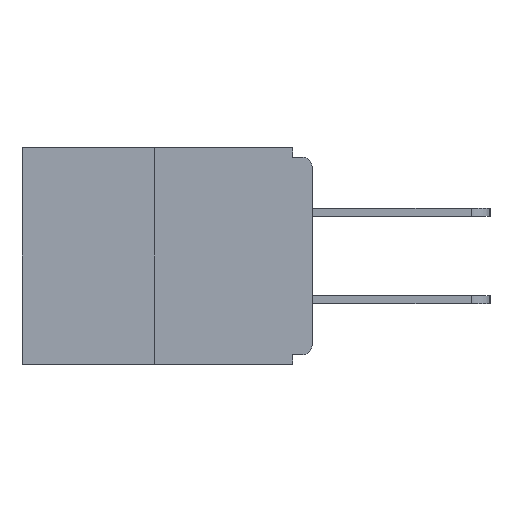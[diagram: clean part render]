
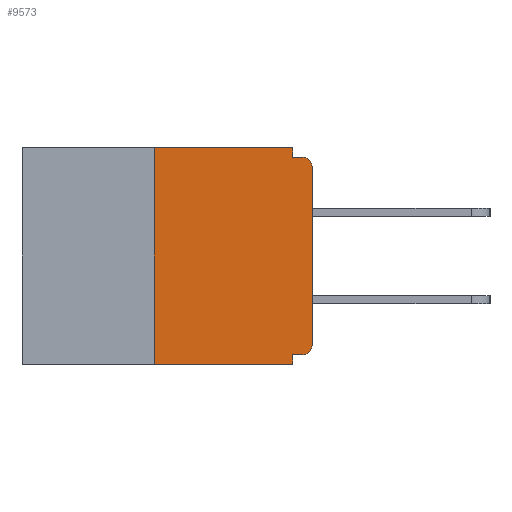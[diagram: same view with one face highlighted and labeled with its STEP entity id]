
A CAD part, left-side view. The second image highlights one B-rep face of the part: STEP entity #9573.
In plain terms, the highlighted planar face has unit normal (-1, 0, 0).
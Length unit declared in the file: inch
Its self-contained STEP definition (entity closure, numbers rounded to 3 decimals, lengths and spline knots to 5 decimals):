
#210 = PLANE ( 'NONE',  #21539 ) ;
#290 = ORIENTED_EDGE ( 'NONE', *, *, #10638, .F. ) ;
#400 = DIRECTION ( 'NONE',  ( 0., 0., 1. ) ) ;
#703 = ORIENTED_EDGE ( 'NONE', *, *, #11095, .T. ) ;
#1531 = CARTESIAN_POINT ( 'NONE',  ( 0., 0., -0.015 ) ) ;
#1739 = ORIENTED_EDGE ( 'NONE', *, *, #9332, .T. ) ;
#2731 = EDGE_CURVE ( 'NONE', #25929, #21995, #11580, .T. ) ;
#2859 = EDGE_CURVE ( 'NONE', #22625, #8743, #8963, .T. ) ;
#3367 = DIRECTION ( 'NONE',  ( 0., -1., 0. ) ) ;
#3566 = VERTEX_POINT ( 'NONE', #13202 ) ;
#4479 = FACE_OUTER_BOUND ( 'NONE', #18576, .T. ) ;
#4932 = VERTEX_POINT ( 'NONE', #13100 ) ;
#5015 = DIRECTION ( 'NONE',  ( 0., 0., -1. ) ) ;
#5588 = ORIENTED_EDGE ( 'NONE', *, *, #16081, .T. ) ;
#5827 = DIRECTION ( 'NONE',  ( 0., 0., -1. ) ) ;
#6580 = ORIENTED_EDGE ( 'NONE', *, *, #21392, .F. ) ;
#6791 = DIRECTION ( 'NONE',  ( -1., 0., 0. ) ) ;
#7643 = VECTOR ( 'NONE', #18172, 39.37008 ) ;
#8652 = CARTESIAN_POINT ( 'NONE',  ( 0., 0.015, -0.015 ) ) ;
#8682 = DIRECTION ( 'NONE',  ( 0., 0., -1. ) ) ;
#8743 = VERTEX_POINT ( 'NONE', #11329 ) ;
#8770 = ORIENTED_EDGE ( 'NONE', *, *, #2859, .F. ) ;
#8963 = LINE ( 'NONE', #15358, #18120 ) ;
#8983 = CARTESIAN_POINT ( 'NONE',  ( 0., 0.031, 0. ) ) ;
#9332 = EDGE_CURVE ( 'NONE', #25929, #12354, #13354, .T. ) ;
#9378 = VECTOR ( 'NONE', #3367, 39.37008 ) ;
#9573 = ADVANCED_FACE ( 'NONE', ( #4479 ), #210, .F. ) ;
#9798 = DIRECTION ( 'NONE',  ( 0., -1., 0. ) ) ;
#9992 = LINE ( 'NONE', #26775, #14894 ) ;
#10056 = DIRECTION ( 'NONE',  ( 0., -1., 0. ) ) ;
#10638 = EDGE_CURVE ( 'NONE', #3566, #10670, #15293, .T. ) ;
#10640 = EDGE_CURVE ( 'NONE', #16415, #3566, #10713, .T. ) ;
#10656 = CARTESIAN_POINT ( 'NONE',  ( 0., 0.015, -0.328 ) ) ;
#10670 = VERTEX_POINT ( 'NONE', #8652 ) ;
#10713 = LINE ( 'NONE', #20143, #14620 ) ;
#11095 = EDGE_CURVE ( 'NONE', #4932, #10670, #24919, .T. ) ;
#11329 = CARTESIAN_POINT ( 'NONE',  ( 0., 0.25, 0. ) ) ;
#11580 = LINE ( 'NONE', #22131, #7643 ) ;
#11700 = AXIS2_PLACEMENT_3D ( 'NONE', #15142, #6791, #23616 ) ;
#12240 = CARTESIAN_POINT ( 'NONE',  ( 0., 0.031, -0.343 ) ) ;
#12354 = VERTEX_POINT ( 'NONE', #24388 ) ;
#12844 = CARTESIAN_POINT ( 'NONE',  ( 0., 0.25, -0.343 ) ) ;
#13100 = CARTESIAN_POINT ( 'NONE',  ( 0., 0., -0.03 ) ) ;
#13164 = CARTESIAN_POINT ( 'NONE',  ( 0., 0.46, 0. ) ) ;
#13202 = CARTESIAN_POINT ( 'NONE',  ( 0., 0.031, -0.015 ) ) ;
#13354 = CIRCLE ( 'NONE', #11700, 0.015 ) ;
#13666 = AXIS2_PLACEMENT_3D ( 'NONE', #17601, #21637, #5015 ) ;
#14080 = CARTESIAN_POINT ( 'NONE',  ( 0., 0.46, -0.343 ) ) ;
#14092 = ORIENTED_EDGE ( 'NONE', *, *, #10640, .F. ) ;
#14620 = VECTOR ( 'NONE', #18119, 39.37008 ) ;
#14894 = VECTOR ( 'NONE', #9798, 39.37008 ) ;
#15142 = CARTESIAN_POINT ( 'NONE',  ( 0., 0.015, -0.313 ) ) ;
#15175 = DIRECTION ( 'NONE',  ( 1., 0., 0. ) ) ;
#15251 = CARTESIAN_POINT ( 'NONE',  ( 0., 0.031, -0.328 ) ) ;
#15293 = LINE ( 'NONE', #1531, #9378 ) ;
#15358 = CARTESIAN_POINT ( 'NONE',  ( 0., 0.25, 0. ) ) ;
#15628 = DIRECTION ( 'NONE',  ( 0., 0., 1. ) ) ;
#16081 = EDGE_CURVE ( 'NONE', #12354, #4932, #17056, .T. ) ;
#16358 = ORIENTED_EDGE ( 'NONE', *, *, #2731, .F. ) ;
#16415 = VERTEX_POINT ( 'NONE', #8983 ) ;
#17056 = LINE ( 'NONE', #25589, #25937 ) ;
#17601 = CARTESIAN_POINT ( 'NONE',  ( 0., 0.015, -0.03 ) ) ;
#17636 = ORIENTED_EDGE ( 'NONE', *, *, #26482, .T. ) ;
#18119 = DIRECTION ( 'NONE',  ( 0., 0., -1. ) ) ;
#18120 = VECTOR ( 'NONE', #15628, 39.37008 ) ;
#18172 = DIRECTION ( 'NONE',  ( 0., 1., 0. ) ) ;
#18576 = EDGE_LOOP ( 'NONE', ( #20257, #8770, #17636, #6580, #16358, #1739, #5588, #703, #290, #14092 ) ) ;
#18770 = EDGE_CURVE ( 'NONE', #8743, #16415, #9992, .T. ) ;
#18992 = VECTOR ( 'NONE', #5827, 39.37008 ) ;
#20143 = CARTESIAN_POINT ( 'NONE',  ( 0., 0.031, 0. ) ) ;
#20257 = ORIENTED_EDGE ( 'NONE', *, *, #18770, .F. ) ;
#20924 = VERTEX_POINT ( 'NONE', #12240 ) ;
#21067 = VECTOR ( 'NONE', #10056, 39.37008 ) ;
#21392 = EDGE_CURVE ( 'NONE', #21995, #20924, #23603, .T. ) ;
#21539 = AXIS2_PLACEMENT_3D ( 'NONE', #13164, #15175, #8682 ) ;
#21637 = DIRECTION ( 'NONE',  ( -1., 0., 0. ) ) ;
#21995 = VERTEX_POINT ( 'NONE', #15251 ) ;
#22131 = CARTESIAN_POINT ( 'NONE',  ( 0., 0., -0.328 ) ) ;
#22625 = VERTEX_POINT ( 'NONE', #12844 ) ;
#23101 = CARTESIAN_POINT ( 'NONE',  ( 0., 0.031, -0.343 ) ) ;
#23603 = LINE ( 'NONE', #23101, #18992 ) ;
#23616 = DIRECTION ( 'NONE',  ( 0., 0., -1. ) ) ;
#24388 = CARTESIAN_POINT ( 'NONE',  ( 0., 0., -0.313 ) ) ;
#24919 = CIRCLE ( 'NONE', #13666, 0.015 ) ;
#25009 = LINE ( 'NONE', #14080, #21067 ) ;
#25589 = CARTESIAN_POINT ( 'NONE',  ( 0., 0., 0. ) ) ;
#25929 = VERTEX_POINT ( 'NONE', #10656 ) ;
#25937 = VECTOR ( 'NONE', #400, 39.37008 ) ;
#26482 = EDGE_CURVE ( 'NONE', #22625, #20924, #25009, .T. ) ;
#26775 = CARTESIAN_POINT ( 'NONE',  ( 0., 0.46, 0. ) ) ;
